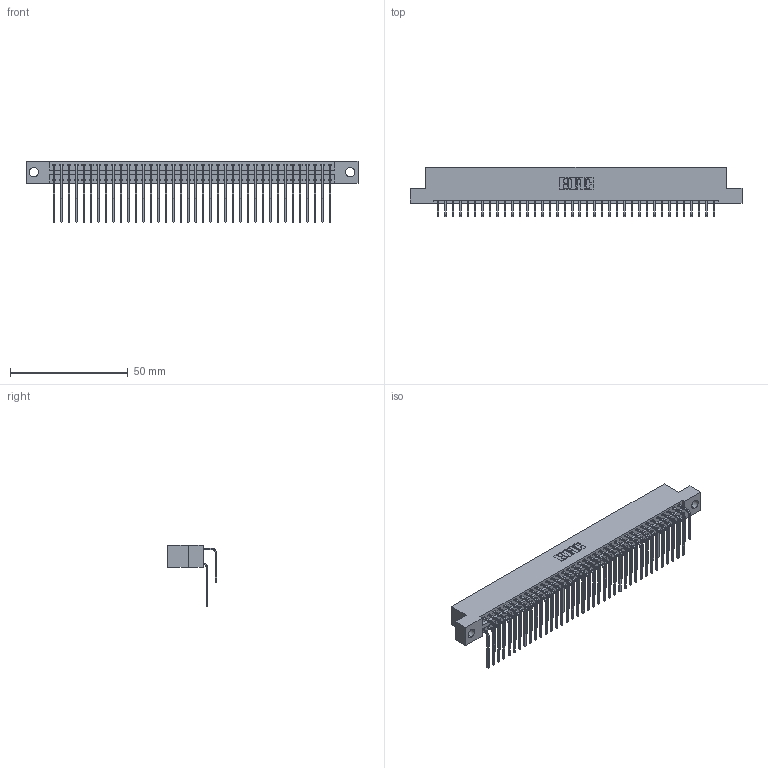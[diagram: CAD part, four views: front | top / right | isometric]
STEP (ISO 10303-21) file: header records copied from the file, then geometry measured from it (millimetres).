
FILE_DESCRIPTION (( 'STEP AP203' ), '1' );
FILE_NAME ('346-076-559-204.STEP', '2018-08-29T04:47:43', ( '' ), ( '' ), 'SwSTEP 2.0', 'SolidWorks 2016', '' );
FILE_SCHEMA (( 'CONFIG_CONTROL_DESIGN' ));
Length unit declared in the file: inch
Products named in the file (4): 346 Part_Flush Mounting Lugs - 0.156 Dia-TH; 345-292-001_558 559 Tail - 1; 345-292-001_559 Tail - 2; 346-076-559-204
Assembly tree (77 placements, depth 2):
  346-076-559-204
    346 Part_Flush Mounting Lugs - 0.156 Dia-TH
    345-292-001_558 559 Tail - 1  x38
    345-292-001_559 Tail - 2  x38
Bounding box: 141.22 x 20.89 x 26.16 mm (x, y, z)
Volume: 14090.6 mm3; surface area: 21222.2 mm2
Topology: 77 solids, 77 shells, 4226 faces, 12565 edges, 8274 vertices
Faces by surface type: plane 2888, cylinder 1338
Entity records: 27125 total; most frequent: CARTESIAN_POINT 4527, ORIENTED_EDGE 4410, DIRECTION 4013, EDGE_CURVE 2205, LINE 1881, VECTOR 1881, VERTEX_POINT 1466, AXIS2_PLACEMENT_3D 1066
